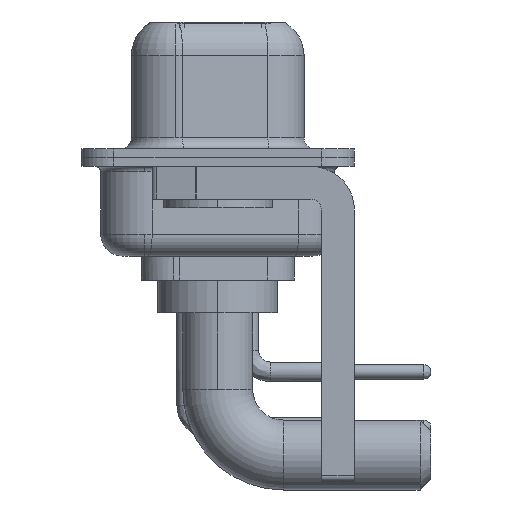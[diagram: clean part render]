
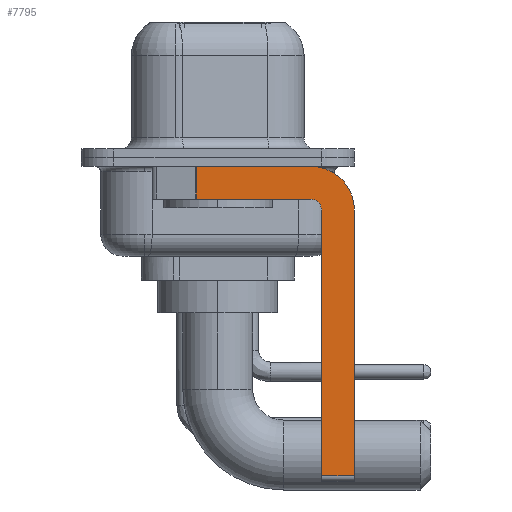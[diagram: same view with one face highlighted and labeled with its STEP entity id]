
A CAD part, left-side view. The second image highlights one B-rep face of the part: STEP entity #7795.
In plain terms, the highlighted planar face has unit normal (-1, 0, 0).
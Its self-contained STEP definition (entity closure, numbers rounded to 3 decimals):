
#110 = CARTESIAN_POINT ( 'NONE',  ( -2.9, -4.25, -1.9 ) ) ;
#237 = DIRECTION ( 'NONE',  ( 0., 0., 1. ) ) ;
#252 = VERTEX_POINT ( 'NONE', #14824 ) ;
#255 = CARTESIAN_POINT ( 'NONE',  ( -2.9, -4.25, -2.4 ) ) ;
#795 = EDGE_CURVE ( 'NONE', #19918, #20071, #17292, .T. ) ;
#1140 = EDGE_CURVE ( 'NONE', #15678, #252, #19134, .T. ) ;
#1671 = CARTESIAN_POINT ( 'NONE',  ( -2.9, -6.25, -14.55 ) ) ;
#2301 = DIRECTION ( 'NONE',  ( 0., -1., 0. ) ) ;
#3303 = FACE_OUTER_BOUND ( 'NONE', #18775, .T. ) ;
#3671 = LINE ( 'NONE', #22591, #9654 ) ;
#3769 = ORIENTED_EDGE ( 'NONE', *, *, #23909, .T. ) ;
#3821 = LINE ( 'NONE', #11502, #18949 ) ;
#4907 = CIRCLE ( 'NONE', #23986, 0.5 ) ;
#5576 = EDGE_CURVE ( 'NONE', #15678, #12194, #3821, .T. ) ;
#5857 = DIRECTION ( 'NONE',  ( 1., 0., 0. ) ) ;
#5907 = DIRECTION ( 'NONE',  ( 0., 0., -1. ) ) ;
#6085 = VERTEX_POINT ( 'NONE', #110 ) ;
#7420 = VECTOR ( 'NONE', #11194, 1000. ) ;
#7795 = ADVANCED_FACE ( 'NONE', ( #3303 ), #16386, .F. ) ;
#8899 = ORIENTED_EDGE ( 'NONE', *, *, #21465, .F. ) ;
#9247 = VECTOR ( 'NONE', #22867, 1000. ) ;
#9360 = AXIS2_PLACEMENT_3D ( 'NONE', #11011, #18504, #22357 ) ;
#9369 = CARTESIAN_POINT ( 'NONE',  ( -2.9, -4.25, -2.4 ) ) ;
#9654 = VECTOR ( 'NONE', #5907, 1000. ) ;
#10971 = ORIENTED_EDGE ( 'NONE', *, *, #1140, .T. ) ;
#11011 = CARTESIAN_POINT ( 'NONE',  ( -2.9, -4.25, -2.4 ) ) ;
#11040 = VECTOR ( 'NONE', #11615, 1000. ) ;
#11194 = DIRECTION ( 'NONE',  ( 0., -1., 0. ) ) ;
#11225 = ORIENTED_EDGE ( 'NONE', *, *, #5576, .F. ) ;
#11311 = AXIS2_PLACEMENT_3D ( 'NONE', #255, #5857, #17068 ) ;
#11432 = CARTESIAN_POINT ( 'NONE',  ( -2.9, 0.978, -0.4 ) ) ;
#11502 = CARTESIAN_POINT ( 'NONE',  ( -2.9, 3., -0.4 ) ) ;
#11615 = DIRECTION ( 'NONE',  ( 0., 0., -1. ) ) ;
#11665 = CARTESIAN_POINT ( 'NONE',  ( -2.9, -4.25, -14.55 ) ) ;
#11737 = LINE ( 'NONE', #15856, #9247 ) ;
#12194 = VERTEX_POINT ( 'NONE', #14952 ) ;
#14824 = CARTESIAN_POINT ( 'NONE',  ( -2.9, 0.978, -1.9 ) ) ;
#14952 = CARTESIAN_POINT ( 'NONE',  ( -2.9, -4.25, -0.4 ) ) ;
#15678 = VERTEX_POINT ( 'NONE', #11432 ) ;
#15856 = CARTESIAN_POINT ( 'NONE',  ( -2.9, -4.25, -1.9 ) ) ;
#16386 = PLANE ( 'NONE',  #9360 ) ;
#16729 = ORIENTED_EDGE ( 'NONE', *, *, #22690, .F. ) ;
#16967 = DIRECTION ( 'NONE',  ( 0., 0., 1. ) ) ;
#17068 = DIRECTION ( 'NONE',  ( 0., 0., -1. ) ) ;
#17292 = LINE ( 'NONE', #19405, #21780 ) ;
#17933 = ORIENTED_EDGE ( 'NONE', *, *, #18708, .F. ) ;
#18088 = CIRCLE ( 'NONE', #11311, 2. ) ;
#18296 = ORIENTED_EDGE ( 'NONE', *, *, #795, .F. ) ;
#18357 = VERTEX_POINT ( 'NONE', #19291 ) ;
#18504 = DIRECTION ( 'NONE',  ( 1., 0., 0. ) ) ;
#18708 = EDGE_CURVE ( 'NONE', #6085, #252, #11737, .T. ) ;
#18775 = EDGE_LOOP ( 'NONE', ( #11225, #10971, #17933, #8899, #18296, #3769, #21768, #16729 ) ) ;
#18949 = VECTOR ( 'NONE', #2301, 1000. ) ;
#19134 = LINE ( 'NONE', #21366, #11040 ) ;
#19195 = EDGE_CURVE ( 'NONE', #18357, #21599, #3671, .T. ) ;
#19291 = CARTESIAN_POINT ( 'NONE',  ( -2.9, -6.25, -2.4 ) ) ;
#19405 = CARTESIAN_POINT ( 'NONE',  ( -2.9, -4.75, -14.8 ) ) ;
#19918 = VERTEX_POINT ( 'NONE', #23620 ) ;
#20071 = VERTEX_POINT ( 'NONE', #20260 ) ;
#20180 = LINE ( 'NONE', #11665, #7420 ) ;
#20260 = CARTESIAN_POINT ( 'NONE',  ( -2.9, -4.75, -2.4 ) ) ;
#21366 = CARTESIAN_POINT ( 'NONE',  ( -2.9, 0.978, -1.9 ) ) ;
#21465 = EDGE_CURVE ( 'NONE', #20071, #6085, #4907, .T. ) ;
#21599 = VERTEX_POINT ( 'NONE', #1671 ) ;
#21768 = ORIENTED_EDGE ( 'NONE', *, *, #19195, .F. ) ;
#21780 = VECTOR ( 'NONE', #237, 1000. ) ;
#22357 = DIRECTION ( 'NONE',  ( 0., 0., -1. ) ) ;
#22591 = CARTESIAN_POINT ( 'NONE',  ( -2.9, -6.25, -2.4 ) ) ;
#22690 = EDGE_CURVE ( 'NONE', #12194, #18357, #18088, .T. ) ;
#22821 = DIRECTION ( 'NONE',  ( -1., 0., 0. ) ) ;
#22867 = DIRECTION ( 'NONE',  ( 0., 1., 0. ) ) ;
#23620 = CARTESIAN_POINT ( 'NONE',  ( -2.9, -4.75, -14.55 ) ) ;
#23909 = EDGE_CURVE ( 'NONE', #19918, #21599, #20180, .T. ) ;
#23986 = AXIS2_PLACEMENT_3D ( 'NONE', #9369, #22821, #16967 ) ;
